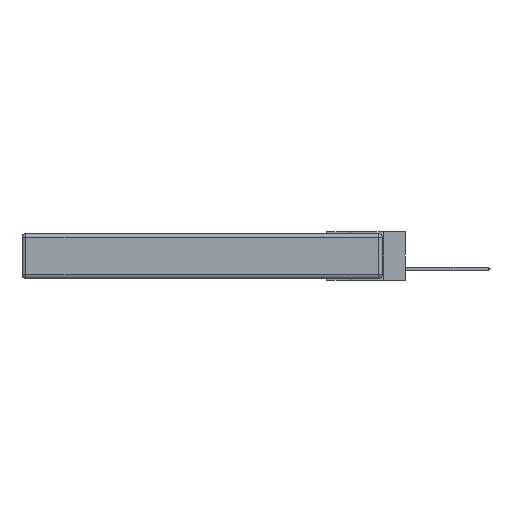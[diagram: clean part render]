
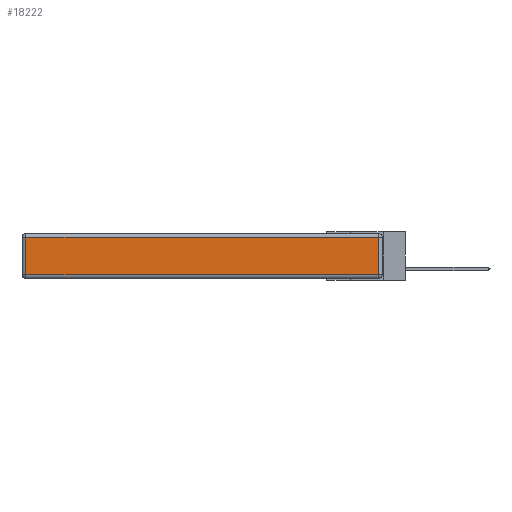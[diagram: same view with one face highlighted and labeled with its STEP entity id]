
A CAD part, left-side view. The second image highlights one B-rep face of the part: STEP entity #18222.
In plain terms, the highlighted planar face has unit normal (-1, 0, 0).
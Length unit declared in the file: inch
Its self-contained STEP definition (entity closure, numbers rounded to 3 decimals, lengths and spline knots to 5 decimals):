
#737 = ORIENTED_EDGE ( 'NONE', *, *, #6480, .T. ) ;
#909 = LINE ( 'NONE', #17383, #26397 ) ;
#4540 = EDGE_CURVE ( 'NONE', #8452, #25964, #909, .T. ) ;
#4550 = ORIENTED_EDGE ( 'NONE', *, *, #5851, .T. ) ;
#4912 = LINE ( 'NONE', #13604, #20459 ) ;
#5690 = VERTEX_POINT ( 'NONE', #13031 ) ;
#5851 = EDGE_CURVE ( 'NONE', #25964, #5690, #12605, .T. ) ;
#6480 = EDGE_CURVE ( 'NONE', #5690, #23742, #23730, .T. ) ;
#6935 = VECTOR ( 'NONE', #25805, 39.37008 ) ;
#7197 = DIRECTION ( 'NONE',  ( 0., 0., 1. ) ) ;
#8452 = VERTEX_POINT ( 'NONE', #17339 ) ;
#8576 = VECTOR ( 'NONE', #13793, 39.37008 ) ;
#8668 = FACE_OUTER_BOUND ( 'NONE', #11302, .T. ) ;
#10206 = DIRECTION ( 'NONE',  ( -1., 0., 0. ) ) ;
#10928 = DIRECTION ( 'NONE',  ( 0., 1., 0. ) ) ;
#11302 = EDGE_LOOP ( 'NONE', ( #737, #19417, #16023, #4550 ) ) ;
#11460 = CARTESIAN_POINT ( 'NONE',  ( 0., 2.72, -0.03 ) ) ;
#12374 = DIRECTION ( 'NONE',  ( 0., 0., 1. ) ) ;
#12605 = LINE ( 'NONE', #21585, #6935 ) ;
#13031 = CARTESIAN_POINT ( 'NONE',  ( 0., 2.72, -0.313 ) ) ;
#13604 = CARTESIAN_POINT ( 'NONE',  ( 0., 0.03, -0.343 ) ) ;
#13793 = DIRECTION ( 'NONE',  ( 0., -1., 0. ) ) ;
#16023 = ORIENTED_EDGE ( 'NONE', *, *, #4540, .T. ) ;
#16504 = CARTESIAN_POINT ( 'NONE',  ( 0., 0., -0.343 ) ) ;
#16811 = CARTESIAN_POINT ( 'NONE',  ( 0., 0.03, -0.313 ) ) ;
#17339 = CARTESIAN_POINT ( 'NONE',  ( 0., 0.03, -0.03 ) ) ;
#17383 = CARTESIAN_POINT ( 'NONE',  ( 0., 2.75, -0.03 ) ) ;
#18222 = ADVANCED_FACE ( 'NONE', ( #8668 ), #22857, .T. ) ;
#19417 = ORIENTED_EDGE ( 'NONE', *, *, #20397, .T. ) ;
#20397 = EDGE_CURVE ( 'NONE', #23742, #8452, #4912, .T. ) ;
#20459 = VECTOR ( 'NONE', #7197, 39.37008 ) ;
#21585 = CARTESIAN_POINT ( 'NONE',  ( 0., 2.72, -0.343 ) ) ;
#22857 = PLANE ( 'NONE',  #25977 ) ;
#23730 = LINE ( 'NONE', #24300, #8576 ) ;
#23742 = VERTEX_POINT ( 'NONE', #16811 ) ;
#24300 = CARTESIAN_POINT ( 'NONE',  ( 0., 0., -0.313 ) ) ;
#25805 = DIRECTION ( 'NONE',  ( 0., 0., -1. ) ) ;
#25964 = VERTEX_POINT ( 'NONE', #11460 ) ;
#25977 = AXIS2_PLACEMENT_3D ( 'NONE', #16504, #10206, #12374 ) ;
#26397 = VECTOR ( 'NONE', #10928, 39.37008 ) ;
